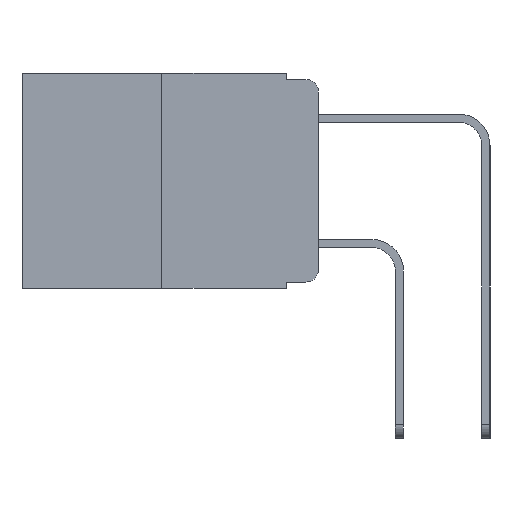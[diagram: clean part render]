
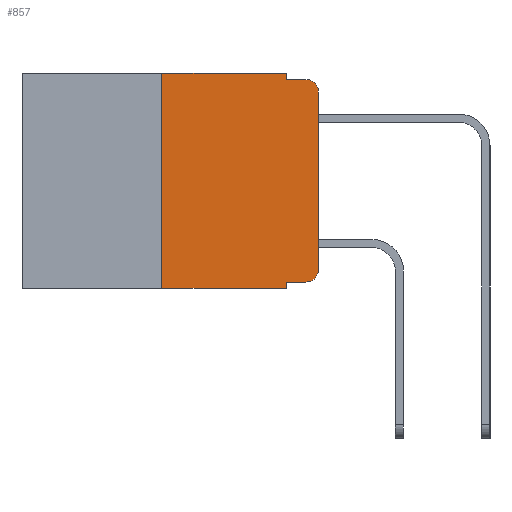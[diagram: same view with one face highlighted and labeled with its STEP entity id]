
A CAD part, left-side view. The second image highlights one B-rep face of the part: STEP entity #857.
In plain terms, the highlighted planar face has unit normal (-1, 0, 0).
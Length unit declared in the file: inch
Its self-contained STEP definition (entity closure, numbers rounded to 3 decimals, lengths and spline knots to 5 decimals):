
#398 = LINE ( 'NONE', #5724, #8973 ) ;
#857 = ADVANCED_FACE ( 'NONE', ( #11232 ), #6869, .F. ) ;
#1008 = DIRECTION ( 'NONE',  ( 0., 0., -1. ) ) ;
#1046 = AXIS2_PLACEMENT_3D ( 'NONE', #10859, #4674, #11869 ) ;
#1151 = VERTEX_POINT ( 'NONE', #1860 ) ;
#1248 = CARTESIAN_POINT ( 'NONE',  ( 0., 0.051, 0. ) ) ;
#1860 = CARTESIAN_POINT ( 'NONE',  ( 0., 0.02, -0.01 ) ) ;
#2043 = VECTOR ( 'NONE', #9043, 39.37008 ) ;
#2125 = DIRECTION ( 'NONE',  ( 0., -1., 0. ) ) ;
#2203 = CARTESIAN_POINT ( 'NONE',  ( 0., 0., -0.03 ) ) ;
#2376 = VERTEX_POINT ( 'NONE', #9577 ) ;
#2665 = EDGE_CURVE ( 'NONE', #10298, #1151, #4746, .T. ) ;
#2829 = EDGE_CURVE ( 'NONE', #8451, #4715, #398, .T. ) ;
#3029 = DIRECTION ( 'NONE',  ( 0., -1., 0. ) ) ;
#3030 = EDGE_CURVE ( 'NONE', #4258, #9771, #3639, .T. ) ;
#3038 = CARTESIAN_POINT ( 'NONE',  ( 0., 0.25, 0. ) ) ;
#3068 = CARTESIAN_POINT ( 'NONE',  ( 0., 0.051, -0.333 ) ) ;
#3157 = ORIENTED_EDGE ( 'NONE', *, *, #5331, .T. ) ;
#3209 = CARTESIAN_POINT ( 'NONE',  ( 0., 0., -0.313 ) ) ;
#3254 = CARTESIAN_POINT ( 'NONE',  ( 0., 0.051, 0. ) ) ;
#3326 = ORIENTED_EDGE ( 'NONE', *, *, #3030, .T. ) ;
#3639 = LINE ( 'NONE', #9928, #11829 ) ;
#3744 = ORIENTED_EDGE ( 'NONE', *, *, #9071, .T. ) ;
#3790 = DIRECTION ( 'NONE',  ( -1., 0., 0. ) ) ;
#4224 = EDGE_LOOP ( 'NONE', ( #3326, #9600, #9069, #6973, #6193, #5878, #4743, #4424, #3744, #3157 ) ) ;
#4258 = VERTEX_POINT ( 'NONE', #3209 ) ;
#4424 = ORIENTED_EDGE ( 'NONE', *, *, #6557, .F. ) ;
#4674 = DIRECTION ( 'NONE',  ( -1., 0., 0. ) ) ;
#4715 = VERTEX_POINT ( 'NONE', #3254 ) ;
#4743 = ORIENTED_EDGE ( 'NONE', *, *, #6715, .T. ) ;
#4746 = LINE ( 'NONE', #12784, #2043 ) ;
#5331 = EDGE_CURVE ( 'NONE', #2376, #4258, #12397, .T. ) ;
#5724 = CARTESIAN_POINT ( 'NONE',  ( 0., 0.473, 0. ) ) ;
#5878 = ORIENTED_EDGE ( 'NONE', *, *, #10871, .F. ) ;
#6070 = DIRECTION ( 'NONE',  ( 1., 0., 0. ) ) ;
#6124 = DIRECTION ( 'NONE',  ( 0., 0., -1. ) ) ;
#6193 = ORIENTED_EDGE ( 'NONE', *, *, #2829, .F. ) ;
#6283 = VERTEX_POINT ( 'NONE', #10092 ) ;
#6323 = CARTESIAN_POINT ( 'NONE',  ( 0., 0.051, 0. ) ) ;
#6447 = CARTESIAN_POINT ( 'NONE',  ( 0., 0.25, -0.343 ) ) ;
#6557 = EDGE_CURVE ( 'NONE', #6283, #6570, #9198, .T. ) ;
#6570 = VERTEX_POINT ( 'NONE', #7438 ) ;
#6715 = EDGE_CURVE ( 'NONE', #10516, #6570, #7933, .T. ) ;
#6849 = CARTESIAN_POINT ( 'NONE',  ( 0., 0.02, -0.313 ) ) ;
#6869 = PLANE ( 'NONE',  #6987 ) ;
#6913 = CARTESIAN_POINT ( 'NONE',  ( 0., 0.473, 0. ) ) ;
#6973 = ORIENTED_EDGE ( 'NONE', *, *, #9255, .F. ) ;
#6987 = AXIS2_PLACEMENT_3D ( 'NONE', #6913, #6070, #6124 ) ;
#7438 = CARTESIAN_POINT ( 'NONE',  ( 0., 0.051, -0.343 ) ) ;
#7933 = LINE ( 'NONE', #11444, #12689 ) ;
#8083 = DIRECTION ( 'NONE',  ( 0., 0., 1. ) ) ;
#8451 = VERTEX_POINT ( 'NONE', #3038 ) ;
#8644 = VECTOR ( 'NONE', #8083, 39.37008 ) ;
#8853 = LINE ( 'NONE', #1248, #12504 ) ;
#8973 = VECTOR ( 'NONE', #2125, 39.37008 ) ;
#8977 = LINE ( 'NONE', #11115, #8644 ) ;
#9043 = DIRECTION ( 'NONE',  ( 0., -1., 0. ) ) ;
#9069 = ORIENTED_EDGE ( 'NONE', *, *, #2665, .F. ) ;
#9071 = EDGE_CURVE ( 'NONE', #6283, #2376, #10472, .T. ) ;
#9198 = LINE ( 'NONE', #6323, #9518 ) ;
#9228 = CARTESIAN_POINT ( 'NONE',  ( 0., 0.051, -0.01 ) ) ;
#9255 = EDGE_CURVE ( 'NONE', #4715, #10298, #8853, .T. ) ;
#9518 = VECTOR ( 'NONE', #9541, 39.37008 ) ;
#9541 = DIRECTION ( 'NONE',  ( 0., 0., -1. ) ) ;
#9577 = CARTESIAN_POINT ( 'NONE',  ( 0., 0.02, -0.333 ) ) ;
#9600 = ORIENTED_EDGE ( 'NONE', *, *, #10679, .T. ) ;
#9771 = VERTEX_POINT ( 'NONE', #2203 ) ;
#9928 = CARTESIAN_POINT ( 'NONE',  ( 0., 0., 0. ) ) ;
#10092 = CARTESIAN_POINT ( 'NONE',  ( 0., 0.051, -0.333 ) ) ;
#10242 = DIRECTION ( 'NONE',  ( 0., -1., 0. ) ) ;
#10298 = VERTEX_POINT ( 'NONE', #9228 ) ;
#10308 = DIRECTION ( 'NONE',  ( 0., 0., 1. ) ) ;
#10472 = LINE ( 'NONE', #3068, #10779 ) ;
#10516 = VERTEX_POINT ( 'NONE', #6447 ) ;
#10679 = EDGE_CURVE ( 'NONE', #9771, #1151, #10905, .T. ) ;
#10779 = VECTOR ( 'NONE', #3029, 39.37008 ) ;
#10859 = CARTESIAN_POINT ( 'NONE',  ( 0., 0.02, -0.03 ) ) ;
#10871 = EDGE_CURVE ( 'NONE', #10516, #8451, #8977, .T. ) ;
#10905 = CIRCLE ( 'NONE', #1046, 0.02 ) ;
#11115 = CARTESIAN_POINT ( 'NONE',  ( 0., 0.25, 0. ) ) ;
#11232 = FACE_OUTER_BOUND ( 'NONE', #4224, .T. ) ;
#11444 = CARTESIAN_POINT ( 'NONE',  ( 0., 0.473, -0.343 ) ) ;
#11548 = DIRECTION ( 'NONE',  ( 0., 0., -1. ) ) ;
#11829 = VECTOR ( 'NONE', #10308, 39.37008 ) ;
#11869 = DIRECTION ( 'NONE',  ( 0., 0., -1. ) ) ;
#12397 = CIRCLE ( 'NONE', #12984, 0.02 ) ;
#12504 = VECTOR ( 'NONE', #11548, 39.37008 ) ;
#12689 = VECTOR ( 'NONE', #10242, 39.37008 ) ;
#12784 = CARTESIAN_POINT ( 'NONE',  ( 0., 0.051, -0.01 ) ) ;
#12984 = AXIS2_PLACEMENT_3D ( 'NONE', #6849, #3790, #1008 ) ;
